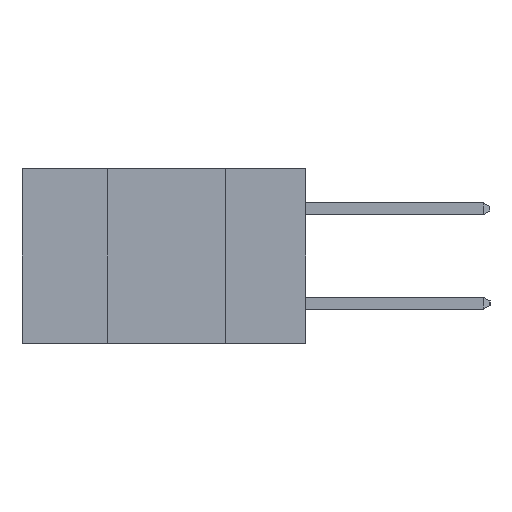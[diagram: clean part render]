
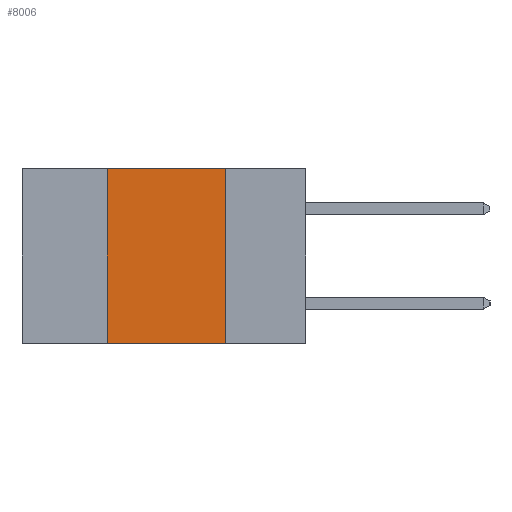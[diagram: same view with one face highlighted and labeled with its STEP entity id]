
A CAD part, left-side view. The second image highlights one B-rep face of the part: STEP entity #8006.
In plain terms, the highlighted planar face has unit normal (-1, 0, 0).
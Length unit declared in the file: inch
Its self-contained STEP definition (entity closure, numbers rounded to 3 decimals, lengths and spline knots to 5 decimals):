
#497 = VERTEX_POINT ( 'NONE', #9701 ) ;
#540 = LINE ( 'NONE', #10795, #12153 ) ;
#931 = ORIENTED_EDGE ( 'NONE', *, *, #5722, .T. ) ;
#1880 = VECTOR ( 'NONE', #10663, 39.37008 ) ;
#2225 = LINE ( 'NONE', #8731, #2566 ) ;
#2566 = VECTOR ( 'NONE', #2725, 39.37008 ) ;
#2680 = CARTESIAN_POINT ( 'NONE',  ( 0., 0.6, 0. ) ) ;
#2725 = DIRECTION ( 'NONE',  ( 0., 0., -1. ) ) ;
#2807 = CARTESIAN_POINT ( 'NONE',  ( 0., 0.42, -0.37 ) ) ;
#3693 = CARTESIAN_POINT ( 'NONE',  ( 0., 0.17, 0. ) ) ;
#3717 = VERTEX_POINT ( 'NONE', #5610 ) ;
#3812 = DIRECTION ( 'NONE',  ( 0., 0., 1. ) ) ;
#3853 = DIRECTION ( 'NONE',  ( 0., -1., 0. ) ) ;
#3966 = PLANE ( 'NONE',  #6704 ) ;
#4970 = DIRECTION ( 'NONE',  ( 1., 0., 0. ) ) ;
#5515 = EDGE_LOOP ( 'NONE', ( #11274, #11501, #5788, #931 ) ) ;
#5610 = CARTESIAN_POINT ( 'NONE',  ( 0., 0.42, 0. ) ) ;
#5615 = EDGE_CURVE ( 'NONE', #11922, #497, #2225, .T. ) ;
#5617 = EDGE_CURVE ( 'NONE', #3717, #11922, #12382, .T. ) ;
#5686 = EDGE_CURVE ( 'NONE', #5694, #3717, #11515, .T. ) ;
#5694 = VERTEX_POINT ( 'NONE', #2807 ) ;
#5722 = EDGE_CURVE ( 'NONE', #5694, #497, #540, .T. ) ;
#5788 = ORIENTED_EDGE ( 'NONE', *, *, #5686, .F. ) ;
#6704 = AXIS2_PLACEMENT_3D ( 'NONE', #7976, #4970, #11821 ) ;
#7976 = CARTESIAN_POINT ( 'NONE',  ( 0., 0.6, 0. ) ) ;
#8006 = ADVANCED_FACE ( 'NONE', ( #12221 ), #3966, .F. ) ;
#8731 = CARTESIAN_POINT ( 'NONE',  ( 0., 0.17, -0.37 ) ) ;
#8814 = CARTESIAN_POINT ( 'NONE',  ( 0., 0.42, -0.37 ) ) ;
#8994 = VECTOR ( 'NONE', #3812, 39.37008 ) ;
#9701 = CARTESIAN_POINT ( 'NONE',  ( 0., 0.17, -0.37 ) ) ;
#10663 = DIRECTION ( 'NONE',  ( 0., -1., 0. ) ) ;
#10795 = CARTESIAN_POINT ( 'NONE',  ( 0., 0.6, -0.37 ) ) ;
#11274 = ORIENTED_EDGE ( 'NONE', *, *, #5615, .F. ) ;
#11501 = ORIENTED_EDGE ( 'NONE', *, *, #5617, .F. ) ;
#11515 = LINE ( 'NONE', #8814, #8994 ) ;
#11821 = DIRECTION ( 'NONE',  ( 0., 0., -1. ) ) ;
#11922 = VERTEX_POINT ( 'NONE', #3693 ) ;
#12153 = VECTOR ( 'NONE', #3853, 39.37008 ) ;
#12221 = FACE_OUTER_BOUND ( 'NONE', #5515, .T. ) ;
#12382 = LINE ( 'NONE', #2680, #1880 ) ;
